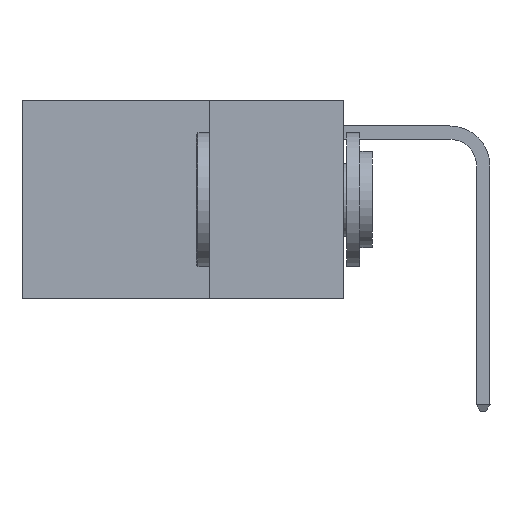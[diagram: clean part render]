
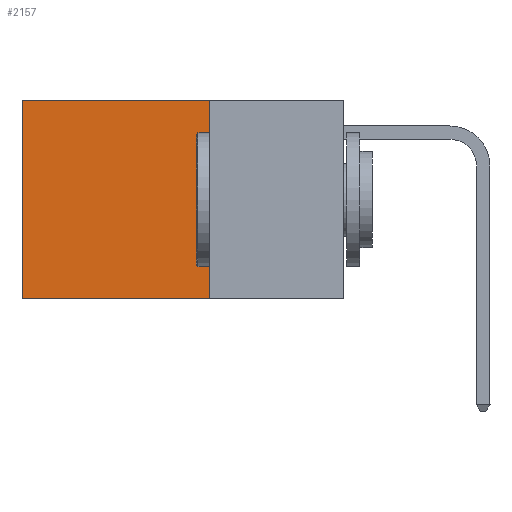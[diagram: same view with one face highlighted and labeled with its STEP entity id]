
A CAD part, left-side view. The second image highlights one B-rep face of the part: STEP entity #2157.
In plain terms, the highlighted planar face has unit normal (-1, 0, 0).
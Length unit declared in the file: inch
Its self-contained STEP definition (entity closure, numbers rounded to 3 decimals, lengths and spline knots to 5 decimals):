
#683 = CARTESIAN_POINT ( 'NONE',  ( 0.2625, 0.25, 0. ) ) ;
#1023 = EDGE_CURVE ( 'NONE', #1605, #2443, #3485, .T. ) ;
#1303 = DIRECTION ( 'NONE',  ( 0., 0., -1. ) ) ;
#1605 = VERTEX_POINT ( 'NONE', #10246 ) ;
#1649 = VERTEX_POINT ( 'NONE', #1812 ) ;
#1812 = CARTESIAN_POINT ( 'NONE',  ( 0.2625, 0.25, -0.37 ) ) ;
#2157 = ADVANCED_FACE ( 'NONE', ( #5299 ), #13214, .F. ) ;
#2334 = LINE ( 'NONE', #3941, #12079 ) ;
#2443 = VERTEX_POINT ( 'NONE', #14435 ) ;
#2864 = EDGE_LOOP ( 'NONE', ( #5332, #4912, #14158, #14113 ) ) ;
#2893 = DIRECTION ( 'NONE',  ( 0., 0., -1. ) ) ;
#3485 = LINE ( 'NONE', #7899, #14450 ) ;
#3803 = CARTESIAN_POINT ( 'NONE',  ( 0.2625, 0.25, 0. ) ) ;
#3941 = CARTESIAN_POINT ( 'NONE',  ( 0.2625, 0.25, -0.37 ) ) ;
#4564 = DIRECTION ( 'NONE',  ( 0., 0., -1. ) ) ;
#4912 = ORIENTED_EDGE ( 'NONE', *, *, #9279, .F. ) ;
#5284 = AXIS2_PLACEMENT_3D ( 'NONE', #7343, #12990, #2893 ) ;
#5294 = DIRECTION ( 'NONE',  ( 0., 1., 0. ) ) ;
#5299 = FACE_OUTER_BOUND ( 'NONE', #2864, .T. ) ;
#5332 = ORIENTED_EDGE ( 'NONE', *, *, #1023, .T. ) ;
#6614 = VECTOR ( 'NONE', #4564, 39.37008 ) ;
#6828 = CARTESIAN_POINT ( 'NONE',  ( 0.2625, 0.25, 0. ) ) ;
#7343 = CARTESIAN_POINT ( 'NONE',  ( 0.2625, 0.25, 0. ) ) ;
#7899 = CARTESIAN_POINT ( 'NONE',  ( 0.2625, 0.6, 0. ) ) ;
#8406 = EDGE_CURVE ( 'NONE', #11726, #1649, #8938, .T. ) ;
#8900 = VECTOR ( 'NONE', #5294, 39.37008 ) ;
#8938 = LINE ( 'NONE', #6828, #6614 ) ;
#9279 = EDGE_CURVE ( 'NONE', #1649, #2443, #2334, .T. ) ;
#9929 = EDGE_CURVE ( 'NONE', #11726, #1605, #13963, .T. ) ;
#10246 = CARTESIAN_POINT ( 'NONE',  ( 0.2625, 0.6, 0. ) ) ;
#11203 = DIRECTION ( 'NONE',  ( 0., 1., 0. ) ) ;
#11726 = VERTEX_POINT ( 'NONE', #3803 ) ;
#12079 = VECTOR ( 'NONE', #11203, 39.37008 ) ;
#12990 = DIRECTION ( 'NONE',  ( 1., 0., 0. ) ) ;
#13214 = PLANE ( 'NONE',  #5284 ) ;
#13963 = LINE ( 'NONE', #683, #8900 ) ;
#14113 = ORIENTED_EDGE ( 'NONE', *, *, #9929, .T. ) ;
#14158 = ORIENTED_EDGE ( 'NONE', *, *, #8406, .F. ) ;
#14435 = CARTESIAN_POINT ( 'NONE',  ( 0.2625, 0.6, -0.37 ) ) ;
#14450 = VECTOR ( 'NONE', #1303, 39.37008 ) ;
